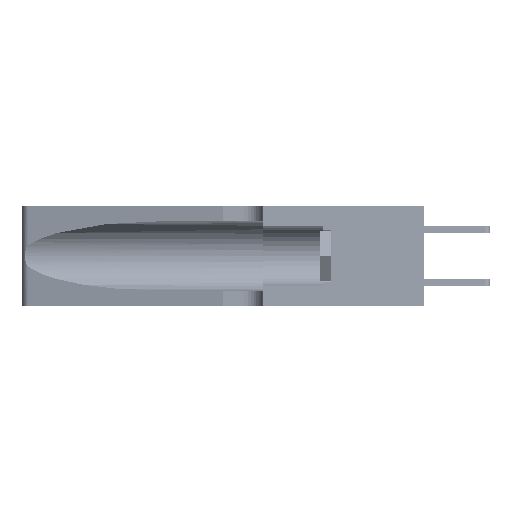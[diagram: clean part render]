
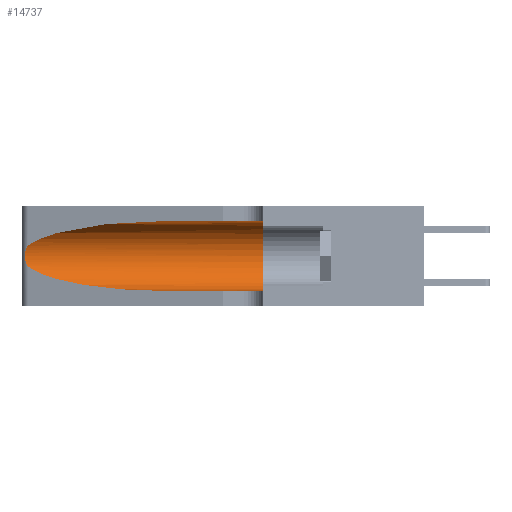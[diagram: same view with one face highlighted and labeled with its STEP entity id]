
A CAD part, left-side view. The second image highlights one B-rep face of the part: STEP entity #14737.
In plain terms, the highlighted cylindrical face has radius 3.308 mm (diameter 6.617 mm), a partial arc.
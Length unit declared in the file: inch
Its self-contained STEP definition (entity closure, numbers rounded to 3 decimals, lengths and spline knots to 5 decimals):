
#24 = VERTEX_POINT ( 'NONE', #12097 ) ;
#1725 = DIRECTION ( 'NONE',  ( 0., 0., -1. ) ) ;
#2066 = EDGE_CURVE ( 'NONE', #24, #35163, #18930, .T. ) ;
#2912 = DIRECTION ( 'NONE',  ( 0., -1., 0. ) ) ;
#3392 = DIRECTION ( 'NONE',  ( 0., -1., 0. ) ) ;
#4059 = CARTESIAN_POINT ( 'NONE',  ( 0.1305, 1.61858, 0.31525 ) ) ;
#5213 = CARTESIAN_POINT ( 'NONE',  ( 0.25789, 1.23486, 0.15765 ) ) ;
#5381 = CARTESIAN_POINT ( 'NONE',  ( 0.1305, 0.72297, 0.05475 ) ) ;
#5883 = CARTESIAN_POINT ( 'NONE',  ( 0.18966, 0.96281, 0.05475 ) ) ;
#6820 = CARTESIAN_POINT ( 'NONE',  ( 0.1305, 0.35, 0.185 ) ) ;
#7066 = CARTESIAN_POINT ( 'NONE',  ( 0.25555, 1.22993, 0.14849 ) ) ;
#7235 = B_SPLINE_CURVE_WITH_KNOTS ( 'NONE', 3,
 ( #31404, #27945, #47725, #14721, #26384, #33828, #33978, #34141, #11745, #34455, #5213, #34605, #7066, #7799 ),
 .UNSPECIFIED., .F., .F.,
 ( 4, 2, 2, 2, 2, 2, 4 ),
 ( 0., 0.00027, 0.00053, 0.00107, 0.0016, 0.00187, 0.00214 ),
 .UNSPECIFIED. ) ;
#7799 = CARTESIAN_POINT ( 'NONE',  ( 0.25487, 1.22718, 0.14631 ) ) ;
#7979 = DIRECTION ( 'NONE',  ( 0., -1., 0. ) ) ;
#8546 = CARTESIAN_POINT ( 'NONE',  ( 0.1305, 0.72297, 0.05475 ) ) ;
#9066 = EDGE_LOOP ( 'NONE', ( #42305, #15938, #18445, #44421, #13312, #25063 ) ) ;
#9348 = AXIS2_PLACEMENT_3D ( 'NONE', #9754, #3392, #1725 ) ;
#9754 = CARTESIAN_POINT ( 'NONE',  ( 0.1305, 1.61858, 0.185 ) ) ;
#11706 = DIRECTION ( 'NONE',  ( 0., 0., 1. ) ) ;
#11745 = CARTESIAN_POINT ( 'NONE',  ( 0.26017, 1.23833, 0.17102 ) ) ;
#12097 = CARTESIAN_POINT ( 'NONE',  ( 0.1305, 0.72297, 0.31525 ) ) ;
#13286 = CARTESIAN_POINT ( 'NONE',  ( 0.25487, 1.22718, 0.22369 ) ) ;
#13312 = ORIENTED_EDGE ( 'NONE', *, *, #44981, .F. ) ;
#13987 = EDGE_CURVE ( 'NONE', #39197, #45597, #7235, .T. ) ;
#14451 = FACE_OUTER_BOUND ( 'NONE', #9066, .T. ) ;
#14721 = CARTESIAN_POINT ( 'NONE',  ( 0.25787, 1.23484, 0.2124 ) ) ;
#14737 = ADVANCED_FACE ( 'NONE', ( #14451 ), #43956, .F. ) ;
#15010 = EDGE_CURVE ( 'NONE', #45597, #21971, #15049, .T. ) ;
#15049 =( BOUNDED_CURVE ( )  B_SPLINE_CURVE ( 3, ( #47200, #24557, #5883, #5381 ),
 .UNSPECIFIED., .F., .F. ) 
 B_SPLINE_CURVE_WITH_KNOTS ( ( 4, 4 ),
 ( 3.44316, 4.71239 ),
 .UNSPECIFIED. ) 
 CURVE ( )  GEOMETRIC_REPRESENTATION_ITEM ( )  RATIONAL_B_SPLINE_CURVE ( ( 1., 0.87, 0.87, 1. ) ) 
 REPRESENTATION_ITEM ( '' )  );
#15938 = ORIENTED_EDGE ( 'NONE', *, *, #13987, .T. ) ;
#18445 = ORIENTED_EDGE ( 'NONE', *, *, #15010, .T. ) ;
#18697 =( BOUNDED_CURVE ( )  B_SPLINE_CURVE ( 3, ( #44878, #29606, #25902, #26230 ),
 .UNSPECIFIED., .F., .F. ) 
 B_SPLINE_CURVE_WITH_KNOTS ( ( 4, 4 ),
 ( 1.5708, 2.84003 ),
 .UNSPECIFIED. ) 
 CURVE ( )  GEOMETRIC_REPRESENTATION_ITEM ( )  RATIONAL_B_SPLINE_CURVE ( ( 1., 0.87, 0.87, 1. ) ) 
 REPRESENTATION_ITEM ( '' )  );
#18930 = LINE ( 'NONE', #4059, #44292 ) ;
#19614 = AXIS2_PLACEMENT_3D ( 'NONE', #6820, #30352, #11706 ) ;
#19907 = VECTOR ( 'NONE', #2912, 39.37008 ) ;
#21098 = EDGE_CURVE ( 'NONE', #21971, #24559, #22225, .T. ) ;
#21971 = VERTEX_POINT ( 'NONE', #8546 ) ;
#22225 = LINE ( 'NONE', #41152, #19907 ) ;
#24557 = CARTESIAN_POINT ( 'NONE',  ( 0.2373, 1.15595, 0.08982 ) ) ;
#24559 = VERTEX_POINT ( 'NONE', #38993 ) ;
#25063 = ORIENTED_EDGE ( 'NONE', *, *, #2066, .F. ) ;
#25902 = CARTESIAN_POINT ( 'NONE',  ( 0.2373, 1.15595, 0.28018 ) ) ;
#26230 = CARTESIAN_POINT ( 'NONE',  ( 0.25487, 1.22718, 0.22369 ) ) ;
#26384 = CARTESIAN_POINT ( 'NONE',  ( 0.25854, 1.2359, 0.20912 ) ) ;
#27945 = CARTESIAN_POINT ( 'NONE',  ( 0.25555, 1.22994, 0.2215 ) ) ;
#28228 = CIRCLE ( 'NONE', #19614, 0.13025 ) ;
#29606 = CARTESIAN_POINT ( 'NONE',  ( 0.18966, 0.96281, 0.31525 ) ) ;
#30141 = CARTESIAN_POINT ( 'NONE',  ( 0.25487, 1.22718, 0.14631 ) ) ;
#30352 = DIRECTION ( 'NONE',  ( 0., 1., 0. ) ) ;
#31404 = CARTESIAN_POINT ( 'NONE',  ( 0.25487, 1.22718, 0.22369 ) ) ;
#33828 = CARTESIAN_POINT ( 'NONE',  ( 0.26018, 1.23835, 0.19895 ) ) ;
#33978 = CARTESIAN_POINT ( 'NONE',  ( 0.26075, 1.23896, 0.19203 ) ) ;
#34141 = CARTESIAN_POINT ( 'NONE',  ( 0.26075, 1.23896, 0.178 ) ) ;
#34455 = CARTESIAN_POINT ( 'NONE',  ( 0.25856, 1.23593, 0.16098 ) ) ;
#34605 = CARTESIAN_POINT ( 'NONE',  ( 0.25639, 1.23186, 0.15144 ) ) ;
#35163 = VERTEX_POINT ( 'NONE', #42929 ) ;
#38993 = CARTESIAN_POINT ( 'NONE',  ( 0.1305, 0.35, 0.05475 ) ) ;
#39197 = VERTEX_POINT ( 'NONE', #13286 ) ;
#41152 = CARTESIAN_POINT ( 'NONE',  ( 0.1305, 1.61858, 0.05475 ) ) ;
#42305 = ORIENTED_EDGE ( 'NONE', *, *, #47193, .T. ) ;
#42929 = CARTESIAN_POINT ( 'NONE',  ( 0.1305, 0.35, 0.31525 ) ) ;
#43956 = CYLINDRICAL_SURFACE ( 'NONE', #9348, 0.13025 ) ;
#44292 = VECTOR ( 'NONE', #7979, 39.37008 ) ;
#44421 = ORIENTED_EDGE ( 'NONE', *, *, #21098, .T. ) ;
#44878 = CARTESIAN_POINT ( 'NONE',  ( 0.1305, 0.72297, 0.31525 ) ) ;
#44981 = EDGE_CURVE ( 'NONE', #35163, #24559, #28228, .T. ) ;
#45597 = VERTEX_POINT ( 'NONE', #30141 ) ;
#47193 = EDGE_CURVE ( 'NONE', #24, #39197, #18697, .T. ) ;
#47200 = CARTESIAN_POINT ( 'NONE',  ( 0.25487, 1.22718, 0.14631 ) ) ;
#47725 = CARTESIAN_POINT ( 'NONE',  ( 0.25639, 1.23184, 0.21858 ) ) ;
